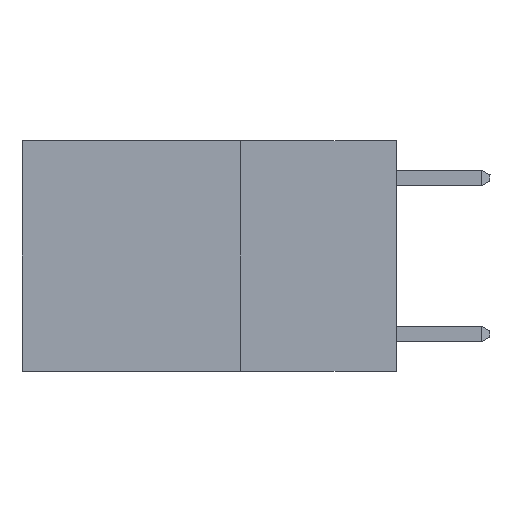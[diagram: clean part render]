
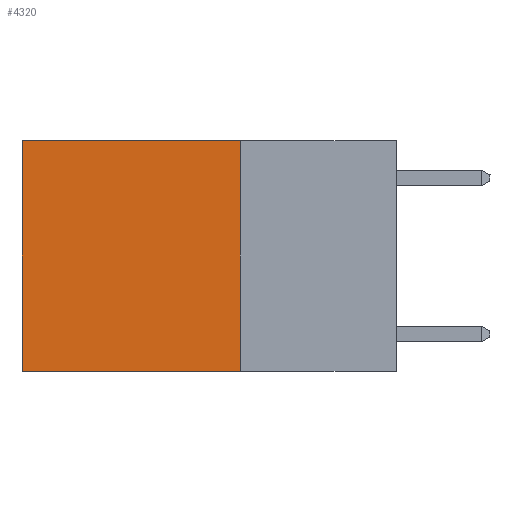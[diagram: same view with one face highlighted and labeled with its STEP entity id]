
A CAD part, left-side view. The second image highlights one B-rep face of the part: STEP entity #4320.
In plain terms, the highlighted planar face has unit normal (-1, 0, 0).
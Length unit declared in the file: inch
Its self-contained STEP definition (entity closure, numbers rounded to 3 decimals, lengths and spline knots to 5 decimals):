
#1196 = LINE ( 'NONE', #2403, #4875 ) ;
#1447 = DIRECTION ( 'NONE',  ( 0., 1., 0. ) ) ;
#1877 = PLANE ( 'NONE',  #7301 ) ;
#1941 = ORIENTED_EDGE ( 'NONE', *, *, #3980, .F. ) ;
#2076 = CARTESIAN_POINT ( 'NONE',  ( 0.2625, 0.25, 0. ) ) ;
#2119 = VERTEX_POINT ( 'NONE', #8353 ) ;
#2403 = CARTESIAN_POINT ( 'NONE',  ( 0.2625, 0.25, 0. ) ) ;
#2740 = CARTESIAN_POINT ( 'NONE',  ( 0.2625, 0.6, -0.37 ) ) ;
#3118 = VECTOR ( 'NONE', #1447, 39.37008 ) ;
#3820 = FACE_OUTER_BOUND ( 'NONE', #4988, .T. ) ;
#3868 = LINE ( 'NONE', #5503, #9926 ) ;
#3980 = EDGE_CURVE ( 'NONE', #8147, #10449, #6207, .T. ) ;
#4154 = LINE ( 'NONE', #7830, #8013 ) ;
#4320 = ADVANCED_FACE ( 'NONE', ( #3820 ), #1877, .F. ) ;
#4875 = VECTOR ( 'NONE', #5008, 39.37008 ) ;
#4988 = EDGE_LOOP ( 'NONE', ( #10977, #1941, #6658, #11964 ) ) ;
#5008 = DIRECTION ( 'NONE',  ( 0., 1., 0. ) ) ;
#5503 = CARTESIAN_POINT ( 'NONE',  ( 0.2625, 0.25, 0. ) ) ;
#5658 = VERTEX_POINT ( 'NONE', #2076 ) ;
#5680 = DIRECTION ( 'NONE',  ( 0., 0., -1. ) ) ;
#6207 = LINE ( 'NONE', #10072, #3118 ) ;
#6658 = ORIENTED_EDGE ( 'NONE', *, *, #10011, .F. ) ;
#6962 = EDGE_CURVE ( 'NONE', #5658, #2119, #1196, .T. ) ;
#7301 = AXIS2_PLACEMENT_3D ( 'NONE', #11492, #7749, #5680 ) ;
#7749 = DIRECTION ( 'NONE',  ( 1., 0., 0. ) ) ;
#7830 = CARTESIAN_POINT ( 'NONE',  ( 0.2625, 0.6, 0. ) ) ;
#7989 = EDGE_CURVE ( 'NONE', #2119, #10449, #4154, .T. ) ;
#8013 = VECTOR ( 'NONE', #11627, 39.37008 ) ;
#8147 = VERTEX_POINT ( 'NONE', #10195 ) ;
#8353 = CARTESIAN_POINT ( 'NONE',  ( 0.2625, 0.6, 0. ) ) ;
#9316 = DIRECTION ( 'NONE',  ( 0., 0., -1. ) ) ;
#9926 = VECTOR ( 'NONE', #9316, 39.37008 ) ;
#10011 = EDGE_CURVE ( 'NONE', #5658, #8147, #3868, .T. ) ;
#10072 = CARTESIAN_POINT ( 'NONE',  ( 0.2625, 0.25, -0.37 ) ) ;
#10195 = CARTESIAN_POINT ( 'NONE',  ( 0.2625, 0.25, -0.37 ) ) ;
#10449 = VERTEX_POINT ( 'NONE', #2740 ) ;
#10977 = ORIENTED_EDGE ( 'NONE', *, *, #7989, .T. ) ;
#11492 = CARTESIAN_POINT ( 'NONE',  ( 0.2625, 0.25, 0. ) ) ;
#11627 = DIRECTION ( 'NONE',  ( 0., 0., -1. ) ) ;
#11964 = ORIENTED_EDGE ( 'NONE', *, *, #6962, .T. ) ;
